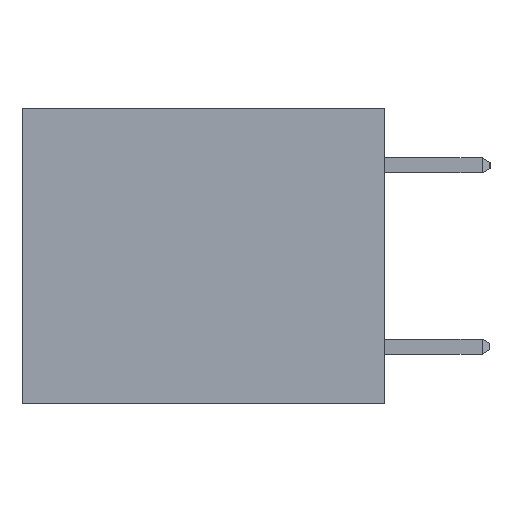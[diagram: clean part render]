
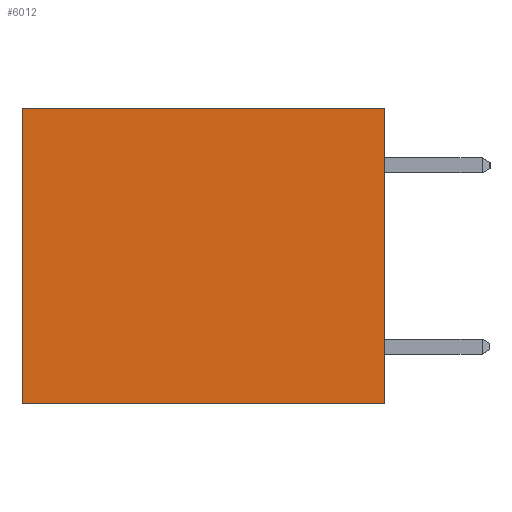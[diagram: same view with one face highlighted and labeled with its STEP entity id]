
A CAD part, left-side view. The second image highlights one B-rep face of the part: STEP entity #6012.
In plain terms, the highlighted planar face has unit normal (-1, 0, 0).
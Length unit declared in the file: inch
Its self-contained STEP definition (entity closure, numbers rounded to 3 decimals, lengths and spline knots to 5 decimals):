
#571 = CARTESIAN_POINT ( 'NONE',  ( 0.3165, 0.6, 0. ) ) ;
#670 = LINE ( 'NONE', #7648, #2244 ) ;
#677 = EDGE_CURVE ( 'NONE', #11363, #1048, #10530, .T. ) ;
#1048 = VERTEX_POINT ( 'NONE', #12812 ) ;
#1278 = FACE_OUTER_BOUND ( 'NONE', #4574, .T. ) ;
#1932 = PLANE ( 'NONE',  #7137 ) ;
#2168 = EDGE_CURVE ( 'NONE', #7586, #6519, #670, .T. ) ;
#2244 = VECTOR ( 'NONE', #9653, 39.37008 ) ;
#2491 = ORIENTED_EDGE ( 'NONE', *, *, #5089, .F. ) ;
#3255 = LINE ( 'NONE', #6632, #12589 ) ;
#3437 = VECTOR ( 'NONE', #8188, 39.37008 ) ;
#4574 = EDGE_LOOP ( 'NONE', ( #7338, #2491, #6802, #6054 ) ) ;
#4823 = LINE ( 'NONE', #10959, #3437 ) ;
#5089 = EDGE_CURVE ( 'NONE', #6519, #1048, #3255, .T. ) ;
#6012 = ADVANCED_FACE ( 'NONE', ( #1278 ), #1932, .F. ) ;
#6054 = ORIENTED_EDGE ( 'NONE', *, *, #6907, .T. ) ;
#6519 = VERTEX_POINT ( 'NONE', #11143 ) ;
#6632 = CARTESIAN_POINT ( 'NONE',  ( 0.3165, 0., -0.49 ) ) ;
#6802 = ORIENTED_EDGE ( 'NONE', *, *, #2168, .F. ) ;
#6907 = EDGE_CURVE ( 'NONE', #7586, #11363, #4823, .T. ) ;
#6937 = CARTESIAN_POINT ( 'NONE',  ( 0.3165, 0., -0.49 ) ) ;
#7137 = AXIS2_PLACEMENT_3D ( 'NONE', #6937, #10906, #9837 ) ;
#7338 = ORIENTED_EDGE ( 'NONE', *, *, #677, .T. ) ;
#7586 = VERTEX_POINT ( 'NONE', #12700 ) ;
#7611 = CARTESIAN_POINT ( 'NONE',  ( 0.3165, 0.6, -0.49 ) ) ;
#7648 = CARTESIAN_POINT ( 'NONE',  ( 0.3165, 0., -0.49 ) ) ;
#8188 = DIRECTION ( 'NONE',  ( 0., 1., 0. ) ) ;
#9145 = VECTOR ( 'NONE', #10515, 39.37008 ) ;
#9653 = DIRECTION ( 'NONE',  ( 0., 0., -1. ) ) ;
#9837 = DIRECTION ( 'NONE',  ( 0., 0., -1. ) ) ;
#10515 = DIRECTION ( 'NONE',  ( 0., 0., -1. ) ) ;
#10530 = LINE ( 'NONE', #7611, #9145 ) ;
#10645 = DIRECTION ( 'NONE',  ( 0., 1., 0. ) ) ;
#10906 = DIRECTION ( 'NONE',  ( 1., 0., 0. ) ) ;
#10959 = CARTESIAN_POINT ( 'NONE',  ( 0.3165, 0., 0. ) ) ;
#11143 = CARTESIAN_POINT ( 'NONE',  ( 0.3165, 0., -0.49 ) ) ;
#11363 = VERTEX_POINT ( 'NONE', #571 ) ;
#12589 = VECTOR ( 'NONE', #10645, 39.37008 ) ;
#12700 = CARTESIAN_POINT ( 'NONE',  ( 0.3165, 0., 0. ) ) ;
#12812 = CARTESIAN_POINT ( 'NONE',  ( 0.3165, 0.6, -0.49 ) ) ;
